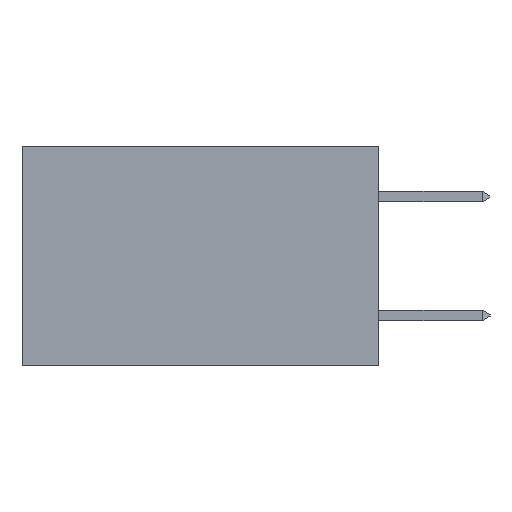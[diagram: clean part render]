
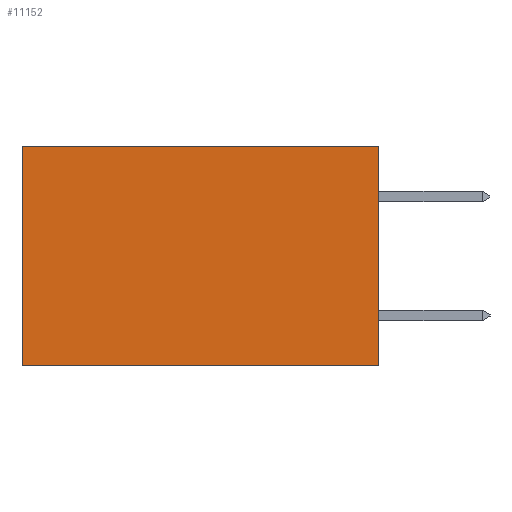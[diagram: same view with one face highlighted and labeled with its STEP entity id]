
A CAD part, left-side view. The second image highlights one B-rep face of the part: STEP entity #11152.
In plain terms, the highlighted planar face has unit normal (-1, 0, 0).
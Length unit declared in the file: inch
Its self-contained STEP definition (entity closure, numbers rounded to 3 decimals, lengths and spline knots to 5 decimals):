
#76 = DIRECTION ( 'NONE',  ( 0., 0., -1. ) ) ;
#461 = LINE ( 'NONE', #10651, #3497 ) ;
#868 = VERTEX_POINT ( 'NONE', #13352 ) ;
#1096 = CARTESIAN_POINT ( 'NONE',  ( 0.2615, 0., 0. ) ) ;
#1119 = AXIS2_PLACEMENT_3D ( 'NONE', #13246, #7111, #76 ) ;
#2200 = EDGE_CURVE ( 'NONE', #14021, #7787, #461, .T. ) ;
#2401 = CARTESIAN_POINT ( 'NONE',  ( 0.2615, 0.6, -0.37 ) ) ;
#3100 = VERTEX_POINT ( 'NONE', #4820 ) ;
#3316 = EDGE_CURVE ( 'NONE', #868, #3100, #12172, .T. ) ;
#3367 = ORIENTED_EDGE ( 'NONE', *, *, #12992, .T. ) ;
#3419 = VECTOR ( 'NONE', #9004, 39.37008 ) ;
#3497 = VECTOR ( 'NONE', #10825, 39.37008 ) ;
#4210 = VECTOR ( 'NONE', #12360, 39.37008 ) ;
#4488 = ORIENTED_EDGE ( 'NONE', *, *, #3316, .F. ) ;
#4820 = CARTESIAN_POINT ( 'NONE',  ( 0.2615, 0., -0.37 ) ) ;
#5042 = PLANE ( 'NONE',  #1119 ) ;
#5676 = EDGE_CURVE ( 'NONE', #3100, #7787, #7600, .T. ) ;
#6013 = LINE ( 'NONE', #1096, #3419 ) ;
#7111 = DIRECTION ( 'NONE',  ( 1., 0., 0. ) ) ;
#7600 = LINE ( 'NONE', #13475, #10418 ) ;
#7787 = VERTEX_POINT ( 'NONE', #2401 ) ;
#9004 = DIRECTION ( 'NONE',  ( 0., 1., 0. ) ) ;
#10341 = EDGE_LOOP ( 'NONE', ( #12661, #11452, #4488, #3367 ) ) ;
#10418 = VECTOR ( 'NONE', #13208, 39.37008 ) ;
#10651 = CARTESIAN_POINT ( 'NONE',  ( 0.2615, 0.6, -0.37 ) ) ;
#10825 = DIRECTION ( 'NONE',  ( 0., 0., -1. ) ) ;
#11152 = ADVANCED_FACE ( 'NONE', ( #13218 ), #5042, .F. ) ;
#11452 = ORIENTED_EDGE ( 'NONE', *, *, #5676, .F. ) ;
#12172 = LINE ( 'NONE', #12417, #4210 ) ;
#12360 = DIRECTION ( 'NONE',  ( 0., 0., -1. ) ) ;
#12394 = CARTESIAN_POINT ( 'NONE',  ( 0.2615, 0.6, 0. ) ) ;
#12417 = CARTESIAN_POINT ( 'NONE',  ( 0.2615, 0., -0.37 ) ) ;
#12661 = ORIENTED_EDGE ( 'NONE', *, *, #2200, .T. ) ;
#12992 = EDGE_CURVE ( 'NONE', #868, #14021, #6013, .T. ) ;
#13208 = DIRECTION ( 'NONE',  ( 0., 1., 0. ) ) ;
#13218 = FACE_OUTER_BOUND ( 'NONE', #10341, .T. ) ;
#13246 = CARTESIAN_POINT ( 'NONE',  ( 0.2615, 0., -0.37 ) ) ;
#13352 = CARTESIAN_POINT ( 'NONE',  ( 0.2615, 0., 0. ) ) ;
#13475 = CARTESIAN_POINT ( 'NONE',  ( 0.2615, 0., -0.37 ) ) ;
#14021 = VERTEX_POINT ( 'NONE', #12394 ) ;
